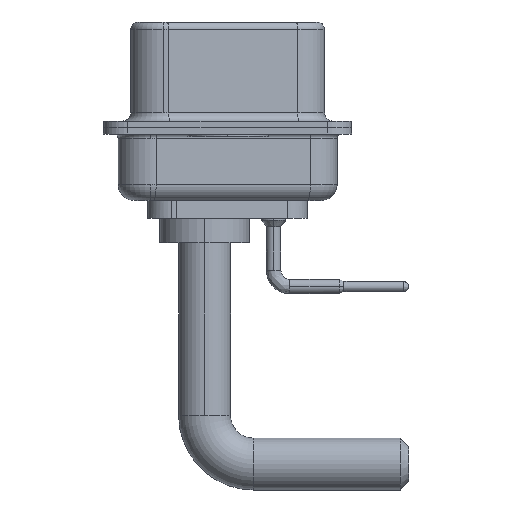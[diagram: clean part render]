
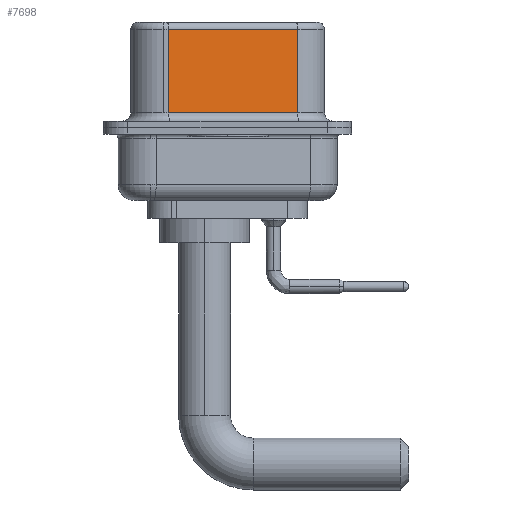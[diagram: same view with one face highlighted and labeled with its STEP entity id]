
A CAD part, left-side view. The second image highlights one B-rep face of the part: STEP entity #7698.
In plain terms, the highlighted planar face has unit normal (-0.985, -0.174, 0).
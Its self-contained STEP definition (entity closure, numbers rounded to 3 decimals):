
#39 = VERTEX_POINT ( 'NONE', #5339 ) ;
#365 = VECTOR ( 'NONE', #12841, 1000. ) ;
#687 = VERTEX_POINT ( 'NONE', #14987 ) ;
#2862 = VECTOR ( 'NONE', #19959, 1000. ) ;
#3117 = VERTEX_POINT ( 'NONE', #17818 ) ;
#3498 = DIRECTION ( 'NONE',  ( 0.985, 0.174, 0. ) ) ;
#4130 = CARTESIAN_POINT ( 'NONE',  ( 3.73, 3.628, 6.52 ) ) ;
#4443 = LINE ( 'NONE', #11249, #18321 ) ;
#5260 = ORIENTED_EDGE ( 'NONE', *, *, #12690, .F. ) ;
#5339 = CARTESIAN_POINT ( 'NONE',  ( 3.73, 3.628, 0.9 ) ) ;
#6144 = LINE ( 'NONE', #14938, #365 ) ;
#7179 = EDGE_CURVE ( 'NONE', #687, #14786, #6144, .T. ) ;
#7698 = ADVANCED_FACE ( 'NONE', ( #12216 ), #19005, .F. ) ;
#8003 = DIRECTION ( 'NONE',  ( 0.174, -0.985, 0. ) ) ;
#8261 = LINE ( 'NONE', #16519, #2862 ) ;
#9053 = DIRECTION ( 'NONE',  ( 0., 0., -1. ) ) ;
#9560 = EDGE_CURVE ( 'NONE', #14786, #39, #14395, .T. ) ;
#10536 = DIRECTION ( 'NONE',  ( -0.174, 0.985, 0. ) ) ;
#11249 = CARTESIAN_POINT ( 'NONE',  ( 5.132, -4.322, 0.9 ) ) ;
#11511 = ORIENTED_EDGE ( 'NONE', *, *, #9560, .T. ) ;
#12216 = FACE_OUTER_BOUND ( 'NONE', #19305, .T. ) ;
#12690 = EDGE_CURVE ( 'NONE', #687, #3117, #8261, .T. ) ;
#12841 = DIRECTION ( 'NONE',  ( -0.174, 0.985, 0. ) ) ;
#14395 = LINE ( 'NONE', #4130, #18761 ) ;
#14786 = VERTEX_POINT ( 'NONE', #21909 ) ;
#14831 = AXIS2_PLACEMENT_3D ( 'NONE', #15442, #3498, #10536 ) ;
#14938 = CARTESIAN_POINT ( 'NONE',  ( 5.132, -4.322, 6.02 ) ) ;
#14987 = CARTESIAN_POINT ( 'NONE',  ( 5.132, -4.322, 6.02 ) ) ;
#15442 = CARTESIAN_POINT ( 'NONE',  ( 5.132, -4.322, 6.52 ) ) ;
#16419 = ORIENTED_EDGE ( 'NONE', *, *, #17916, .T. ) ;
#16519 = CARTESIAN_POINT ( 'NONE',  ( 5.132, -4.322, 6.52 ) ) ;
#17818 = CARTESIAN_POINT ( 'NONE',  ( 5.132, -4.322, 0.9 ) ) ;
#17916 = EDGE_CURVE ( 'NONE', #39, #3117, #4443, .T. ) ;
#18321 = VECTOR ( 'NONE', #8003, 1000. ) ;
#18761 = VECTOR ( 'NONE', #9053, 1000. ) ;
#19005 = PLANE ( 'NONE',  #14831 ) ;
#19305 = EDGE_LOOP ( 'NONE', ( #5260, #20324, #11511, #16419 ) ) ;
#19959 = DIRECTION ( 'NONE',  ( 0., 0., -1. ) ) ;
#20324 = ORIENTED_EDGE ( 'NONE', *, *, #7179, .T. ) ;
#21909 = CARTESIAN_POINT ( 'NONE',  ( 3.73, 3.628, 6.02 ) ) ;
